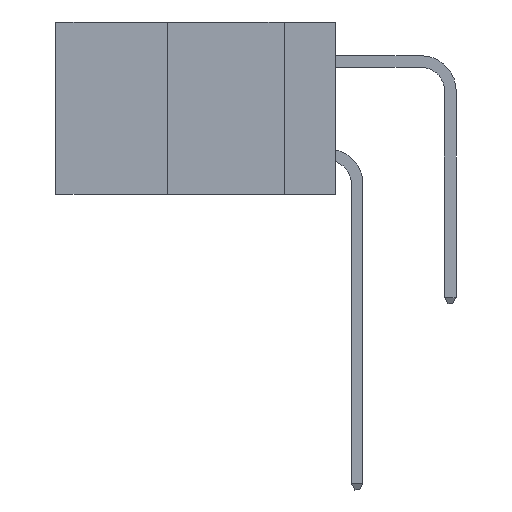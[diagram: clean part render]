
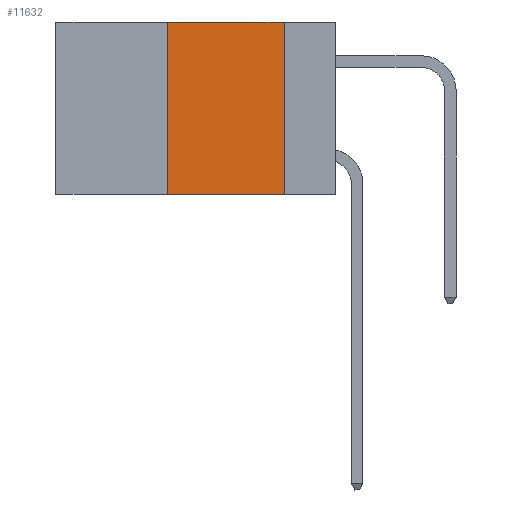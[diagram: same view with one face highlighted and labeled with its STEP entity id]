
A CAD part, left-side view. The second image highlights one B-rep face of the part: STEP entity #11632.
In plain terms, the highlighted planar face has unit normal (-1, 0, 0).
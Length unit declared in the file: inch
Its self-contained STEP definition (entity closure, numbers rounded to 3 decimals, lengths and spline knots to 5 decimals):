
#330 = CARTESIAN_POINT ( 'NONE',  ( 0., 0.6, 0. ) ) ;
#345 = LINE ( 'NONE', #5460, #8123 ) ;
#705 = VECTOR ( 'NONE', #1994, 39.37008 ) ;
#1218 = DIRECTION ( 'NONE',  ( 0., -1., 0. ) ) ;
#1809 = ORIENTED_EDGE ( 'NONE', *, *, #8001, .F. ) ;
#1972 = AXIS2_PLACEMENT_3D ( 'NONE', #3516, #6239, #7015 ) ;
#1994 = DIRECTION ( 'NONE',  ( 0., 0., 1. ) ) ;
#2554 = ORIENTED_EDGE ( 'NONE', *, *, #10361, .F. ) ;
#2597 = DIRECTION ( 'NONE',  ( 0., 0., -1. ) ) ;
#2640 = CARTESIAN_POINT ( 'NONE',  ( 0., 0.11, 0. ) ) ;
#3212 = EDGE_CURVE ( 'NONE', #7174, #8018, #7369, .T. ) ;
#3505 = CARTESIAN_POINT ( 'NONE',  ( 0., 0.36, -0.37 ) ) ;
#3516 = CARTESIAN_POINT ( 'NONE',  ( 0., 0.6, 0. ) ) ;
#3678 = CARTESIAN_POINT ( 'NONE',  ( 0., 0.36, 0. ) ) ;
#4393 = CARTESIAN_POINT ( 'NONE',  ( 0., 0.11, -0.37 ) ) ;
#4869 = CARTESIAN_POINT ( 'NONE',  ( 0., 0.36, 0. ) ) ;
#5460 = CARTESIAN_POINT ( 'NONE',  ( 0., 0.11, 0. ) ) ;
#5605 = ORIENTED_EDGE ( 'NONE', *, *, #3212, .T. ) ;
#5748 = FACE_OUTER_BOUND ( 'NONE', #7743, .T. ) ;
#6239 = DIRECTION ( 'NONE',  ( 1., 0., 0. ) ) ;
#7015 = DIRECTION ( 'NONE',  ( 0., 0., -1. ) ) ;
#7174 = VERTEX_POINT ( 'NONE', #3505 ) ;
#7369 = LINE ( 'NONE', #11639, #10767 ) ;
#7482 = LINE ( 'NONE', #330, #9727 ) ;
#7743 = EDGE_LOOP ( 'NONE', ( #1809, #2554, #9278, #5605 ) ) ;
#8001 = EDGE_CURVE ( 'NONE', #8102, #8018, #345, .T. ) ;
#8018 = VERTEX_POINT ( 'NONE', #4393 ) ;
#8102 = VERTEX_POINT ( 'NONE', #2640 ) ;
#8123 = VECTOR ( 'NONE', #2597, 39.37008 ) ;
#8154 = DIRECTION ( 'NONE',  ( 0., -1., 0. ) ) ;
#8316 = VERTEX_POINT ( 'NONE', #4869 ) ;
#9278 = ORIENTED_EDGE ( 'NONE', *, *, #10222, .F. ) ;
#9727 = VECTOR ( 'NONE', #1218, 39.37008 ) ;
#9895 = PLANE ( 'NONE',  #1972 ) ;
#10222 = EDGE_CURVE ( 'NONE', #7174, #8316, #10299, .T. ) ;
#10299 = LINE ( 'NONE', #3678, #705 ) ;
#10361 = EDGE_CURVE ( 'NONE', #8316, #8102, #7482, .T. ) ;
#10767 = VECTOR ( 'NONE', #8154, 39.37008 ) ;
#11632 = ADVANCED_FACE ( 'NONE', ( #5748 ), #9895, .F. ) ;
#11639 = CARTESIAN_POINT ( 'NONE',  ( 0., 0.6, -0.37 ) ) ;
